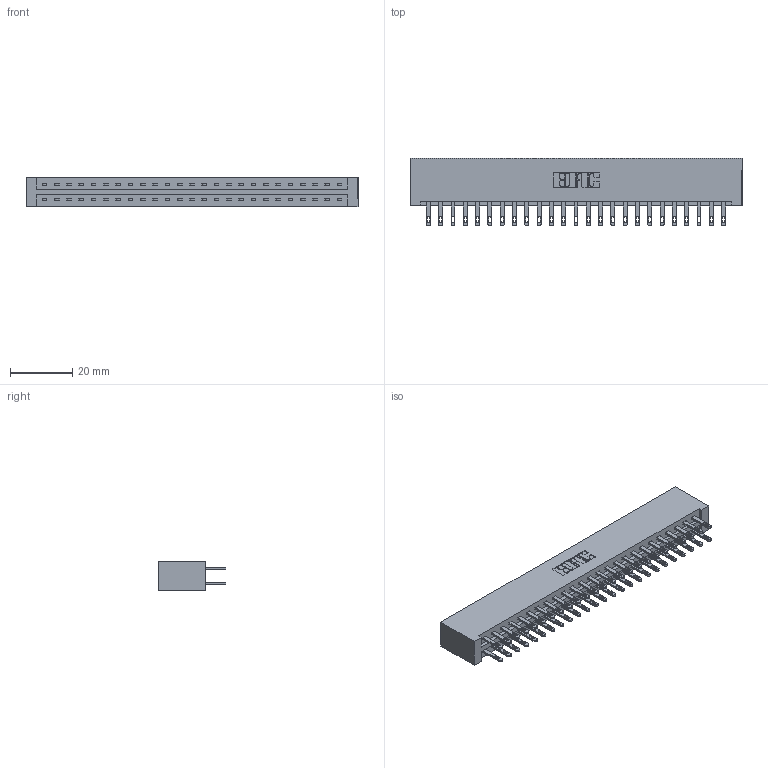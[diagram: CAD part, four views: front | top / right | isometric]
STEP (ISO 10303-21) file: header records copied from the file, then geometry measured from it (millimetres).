
FILE_DESCRIPTION (( 'STEP AP203' ), '1' );
FILE_NAME ('337-050-500-201.STEP', '2019-10-09T15:23:25', ( '' ), ( '' ), 'SwSTEP 2.0', 'SolidWorks 2016', '' );
FILE_SCHEMA (( 'CONFIG_CONTROL_DESIGN' ));
Length unit declared in the file: inch
Products named in the file (3): 337 Part_No Mounting Lugs; 337-050-500-201; 345-292-001_345-293-100
Assembly tree (51 placements, depth 2):
  337-050-500-201
    337 Part_No Mounting Lugs
    345-292-001_345-293-100  x50
Bounding box: 106.93 x 21.85 x 9.4 mm (x, y, z)
Volume: 11956.8 mm3; surface area: 13962.9 mm2
Topology: 51 solids, 51 shells, 2606 faces, 7937 edges, 5290 vertices
Faces by surface type: plane 1666, cylinder 940
Entity records: 21235 total; most frequent: CARTESIAN_POINT 3590, ORIENTED_EDGE 3526, DIRECTION 3079, EDGE_CURVE 1763, VECTOR 1639, LINE 1639, VERTEX_POINT 1174, AXIS2_PLACEMENT_3D 720
